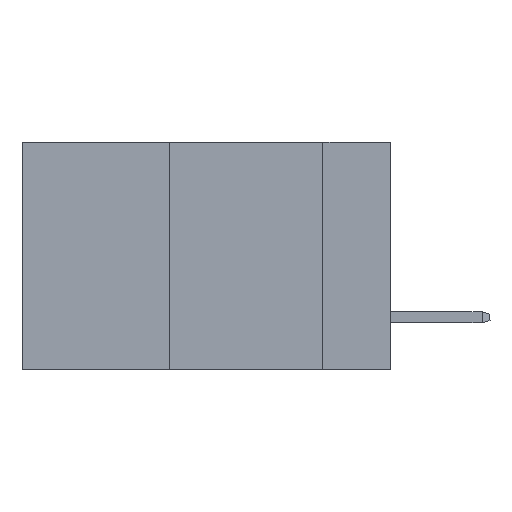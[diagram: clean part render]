
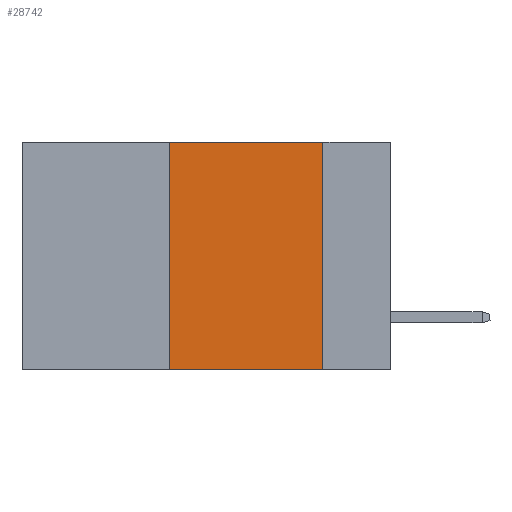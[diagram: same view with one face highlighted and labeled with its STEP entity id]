
A CAD part, left-side view. The second image highlights one B-rep face of the part: STEP entity #28742.
In plain terms, the highlighted planar face has unit normal (-1, 0, 0).
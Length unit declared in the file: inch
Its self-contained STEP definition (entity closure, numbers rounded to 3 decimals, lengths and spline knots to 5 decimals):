
#45 = CARTESIAN_POINT ( 'NONE',  ( 0., 0.11, 0. ) ) ;
#52 = VECTOR ( 'NONE', #18981, 39.37008 ) ;
#2020 = VERTEX_POINT ( 'NONE', #24936 ) ;
#3387 = EDGE_CURVE ( 'NONE', #20555, #8362, #18872, .T. ) ;
#3564 = VECTOR ( 'NONE', #16146, 39.37008 ) ;
#3988 = EDGE_CURVE ( 'NONE', #20555, #2020, #14470, .T. ) ;
#4563 = CARTESIAN_POINT ( 'NONE',  ( 0., 0.6, -0.37 ) ) ;
#5812 = CARTESIAN_POINT ( 'NONE',  ( 0., 0.36, -0.37 ) ) ;
#6554 = ORIENTED_EDGE ( 'NONE', *, *, #3387, .F. ) ;
#7902 = LINE ( 'NONE', #45, #25927 ) ;
#8362 = VERTEX_POINT ( 'NONE', #28151 ) ;
#8715 = CARTESIAN_POINT ( 'NONE',  ( 0., 0.6, 0. ) ) ;
#8965 = EDGE_CURVE ( 'NONE', #8362, #14883, #12607, .T. ) ;
#11125 = PLANE ( 'NONE',  #13355 ) ;
#11408 = CARTESIAN_POINT ( 'NONE',  ( 0., 0.6, 0. ) ) ;
#12607 = LINE ( 'NONE', #11408, #3564 ) ;
#13038 = EDGE_LOOP ( 'NONE', ( #23160, #18354, #6554, #25338 ) ) ;
#13355 = AXIS2_PLACEMENT_3D ( 'NONE', #8715, #13470, #29892 ) ;
#13470 = DIRECTION ( 'NONE',  ( 1., 0., 0. ) ) ;
#13871 = FACE_OUTER_BOUND ( 'NONE', #13038, .T. ) ;
#14470 = LINE ( 'NONE', #4563, #26937 ) ;
#14883 = VERTEX_POINT ( 'NONE', #20711 ) ;
#16146 = DIRECTION ( 'NONE',  ( 0., -1., 0. ) ) ;
#18354 = ORIENTED_EDGE ( 'NONE', *, *, #8965, .F. ) ;
#18790 = CARTESIAN_POINT ( 'NONE',  ( 0., 0.36, 0. ) ) ;
#18872 = LINE ( 'NONE', #18790, #52 ) ;
#18981 = DIRECTION ( 'NONE',  ( 0., 0., 1. ) ) ;
#20555 = VERTEX_POINT ( 'NONE', #5812 ) ;
#20711 = CARTESIAN_POINT ( 'NONE',  ( 0., 0.11, 0. ) ) ;
#23160 = ORIENTED_EDGE ( 'NONE', *, *, #24124, .F. ) ;
#23326 = DIRECTION ( 'NONE',  ( 0., -1., 0. ) ) ;
#23606 = DIRECTION ( 'NONE',  ( 0., 0., -1. ) ) ;
#24124 = EDGE_CURVE ( 'NONE', #14883, #2020, #7902, .T. ) ;
#24936 = CARTESIAN_POINT ( 'NONE',  ( 0., 0.11, -0.37 ) ) ;
#25338 = ORIENTED_EDGE ( 'NONE', *, *, #3988, .T. ) ;
#25927 = VECTOR ( 'NONE', #23606, 39.37008 ) ;
#26937 = VECTOR ( 'NONE', #23326, 39.37008 ) ;
#28151 = CARTESIAN_POINT ( 'NONE',  ( 0., 0.36, 0. ) ) ;
#28742 = ADVANCED_FACE ( 'NONE', ( #13871 ), #11125, .F. ) ;
#29892 = DIRECTION ( 'NONE',  ( 0., 0., -1. ) ) ;
